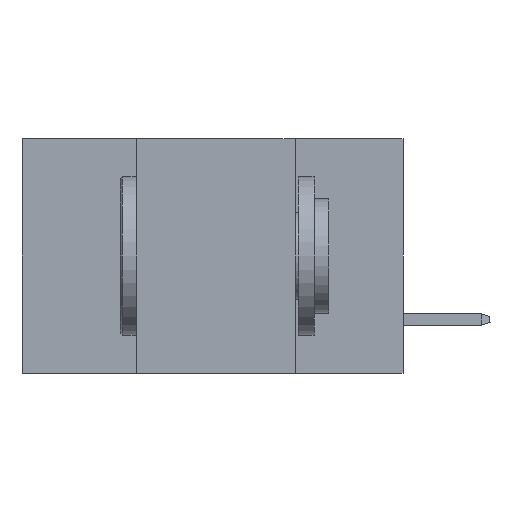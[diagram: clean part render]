
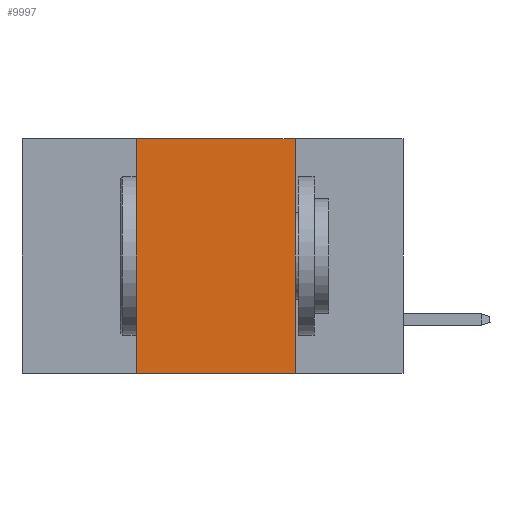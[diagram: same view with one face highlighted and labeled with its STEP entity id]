
A CAD part, left-side view. The second image highlights one B-rep face of the part: STEP entity #9997.
In plain terms, the highlighted planar face has unit normal (-1, 0, 0).
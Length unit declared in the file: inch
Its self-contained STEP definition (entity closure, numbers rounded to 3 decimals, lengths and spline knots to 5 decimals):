
#72 = CARTESIAN_POINT ( 'NONE',  ( 0., 0.42, 0. ) ) ;
#1228 = LINE ( 'NONE', #10531, #9723 ) ;
#2304 = VERTEX_POINT ( 'NONE', #72 ) ;
#4866 = CARTESIAN_POINT ( 'NONE',  ( 0., 0.6, 0. ) ) ;
#4930 = VERTEX_POINT ( 'NONE', #26966 ) ;
#5357 = CARTESIAN_POINT ( 'NONE',  ( 0., 0.42, 0. ) ) ;
#5498 = ORIENTED_EDGE ( 'NONE', *, *, #12216, .F. ) ;
#5978 = CARTESIAN_POINT ( 'NONE',  ( 0., 0.6, -0.37 ) ) ;
#9354 = DIRECTION ( 'NONE',  ( 0., 0., -1. ) ) ;
#9723 = VECTOR ( 'NONE', #14841, 39.37008 ) ;
#9960 = VECTOR ( 'NONE', #24241, 39.37008 ) ;
#9997 = ADVANCED_FACE ( 'NONE', ( #23598 ), #11841, .F. ) ;
#10531 = CARTESIAN_POINT ( 'NONE',  ( 0., 0.6, 0. ) ) ;
#11841 = PLANE ( 'NONE',  #18707 ) ;
#12216 = EDGE_CURVE ( 'NONE', #19409, #4930, #17260, .T. ) ;
#14446 = VECTOR ( 'NONE', #23951, 39.37008 ) ;
#14465 = DIRECTION ( 'NONE',  ( 1., 0., 0. ) ) ;
#14841 = DIRECTION ( 'NONE',  ( 0., -1., 0. ) ) ;
#14961 = ORIENTED_EDGE ( 'NONE', *, *, #28984, .T. ) ;
#15388 = LINE ( 'NONE', #5978, #9960 ) ;
#17110 = CARTESIAN_POINT ( 'NONE',  ( 0., 0.17, 0. ) ) ;
#17260 = LINE ( 'NONE', #17110, #19264 ) ;
#18707 = AXIS2_PLACEMENT_3D ( 'NONE', #4866, #14465, #9354 ) ;
#18992 = CARTESIAN_POINT ( 'NONE',  ( 0., 0.42, -0.37 ) ) ;
#19264 = VECTOR ( 'NONE', #22363, 39.37008 ) ;
#19409 = VERTEX_POINT ( 'NONE', #21013 ) ;
#21013 = CARTESIAN_POINT ( 'NONE',  ( 0., 0.17, 0. ) ) ;
#21997 = EDGE_CURVE ( 'NONE', #2304, #19409, #1228, .T. ) ;
#22363 = DIRECTION ( 'NONE',  ( 0., 0., -1. ) ) ;
#23304 = ORIENTED_EDGE ( 'NONE', *, *, #21997, .F. ) ;
#23598 = FACE_OUTER_BOUND ( 'NONE', #27252, .T. ) ;
#23951 = DIRECTION ( 'NONE',  ( 0., 0., 1. ) ) ;
#24241 = DIRECTION ( 'NONE',  ( 0., -1., 0. ) ) ;
#26563 = LINE ( 'NONE', #5357, #14446 ) ;
#26966 = CARTESIAN_POINT ( 'NONE',  ( 0., 0.17, -0.37 ) ) ;
#27252 = EDGE_LOOP ( 'NONE', ( #5498, #23304, #28471, #14961 ) ) ;
#28471 = ORIENTED_EDGE ( 'NONE', *, *, #30194, .F. ) ;
#28924 = VERTEX_POINT ( 'NONE', #18992 ) ;
#28984 = EDGE_CURVE ( 'NONE', #28924, #4930, #15388, .T. ) ;
#30194 = EDGE_CURVE ( 'NONE', #28924, #2304, #26563, .T. ) ;
